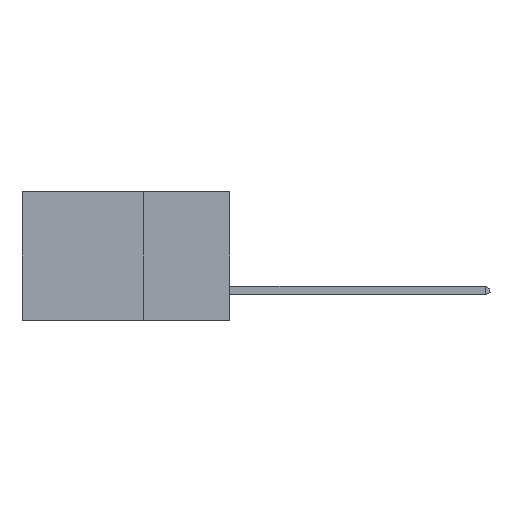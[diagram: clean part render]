
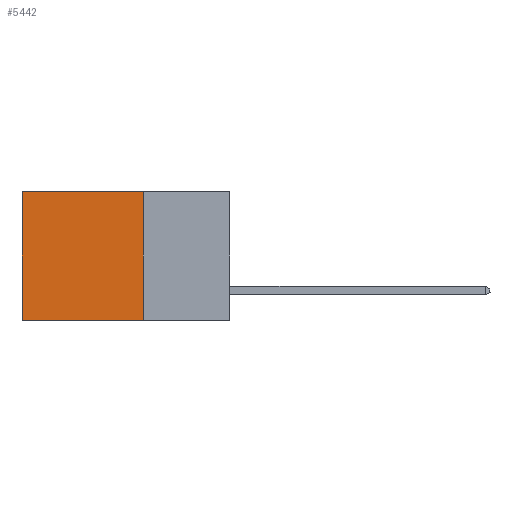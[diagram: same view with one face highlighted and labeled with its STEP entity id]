
A CAD part, left-side view. The second image highlights one B-rep face of the part: STEP entity #5442.
In plain terms, the highlighted planar face has unit normal (-1, 0, 0).
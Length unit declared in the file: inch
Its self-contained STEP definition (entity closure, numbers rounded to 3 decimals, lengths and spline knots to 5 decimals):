
#1410 = ORIENTED_EDGE ( 'NONE', *, *, #19259, .F. ) ;
#1640 = FACE_OUTER_BOUND ( 'NONE', #2733, .T. ) ;
#1818 = LINE ( 'NONE', #10269, #3425 ) ;
#2164 = VERTEX_POINT ( 'NONE', #7322 ) ;
#2174 = LINE ( 'NONE', #19444, #2698 ) ;
#2231 = ORIENTED_EDGE ( 'NONE', *, *, #9099, .T. ) ;
#2688 = PLANE ( 'NONE',  #17670 ) ;
#2698 = VECTOR ( 'NONE', #7493, 39.37008 ) ;
#2733 = EDGE_LOOP ( 'NONE', ( #9293, #13278, #1410, #2231 ) ) ;
#2766 = DIRECTION ( 'NONE',  ( 1., 0., 0. ) ) ;
#2942 = CARTESIAN_POINT ( 'NONE',  ( 0.298, 0.25, 0. ) ) ;
#3425 = VECTOR ( 'NONE', #22427, 39.37008 ) ;
#3997 = DIRECTION ( 'NONE',  ( 0., 1., 0. ) ) ;
#4279 = EDGE_CURVE ( 'NONE', #2164, #12227, #11445, .T. ) ;
#5243 = VECTOR ( 'NONE', #5940, 39.37008 ) ;
#5442 = ADVANCED_FACE ( 'NONE', ( #1640 ), #2688, .F. ) ;
#5940 = DIRECTION ( 'NONE',  ( 0., 1., 0. ) ) ;
#7322 = CARTESIAN_POINT ( 'NONE',  ( 0.298, 0.25, -0.37 ) ) ;
#7493 = DIRECTION ( 'NONE',  ( 0., 0., -1. ) ) ;
#9099 = EDGE_CURVE ( 'NONE', #9433, #19829, #12307, .T. ) ;
#9228 = CARTESIAN_POINT ( 'NONE',  ( 0.298, 0.6, 0. ) ) ;
#9293 = ORIENTED_EDGE ( 'NONE', *, *, #10940, .T. ) ;
#9433 = VERTEX_POINT ( 'NONE', #2942 ) ;
#10146 = CARTESIAN_POINT ( 'NONE',  ( 0.298, 0.6, -0.37 ) ) ;
#10269 = CARTESIAN_POINT ( 'NONE',  ( 0.298, 0.25, 0. ) ) ;
#10940 = EDGE_CURVE ( 'NONE', #19829, #12227, #2174, .T. ) ;
#11239 = CARTESIAN_POINT ( 'NONE',  ( 0.298, 0.25, 0. ) ) ;
#11445 = LINE ( 'NONE', #21309, #20142 ) ;
#12227 = VERTEX_POINT ( 'NONE', #10146 ) ;
#12307 = LINE ( 'NONE', #12435, #5243 ) ;
#12435 = CARTESIAN_POINT ( 'NONE',  ( 0.298, 0.25, 0. ) ) ;
#13278 = ORIENTED_EDGE ( 'NONE', *, *, #4279, .F. ) ;
#17670 = AXIS2_PLACEMENT_3D ( 'NONE', #11239, #2766, #19980 ) ;
#19259 = EDGE_CURVE ( 'NONE', #9433, #2164, #1818, .T. ) ;
#19444 = CARTESIAN_POINT ( 'NONE',  ( 0.298, 0.6, 0. ) ) ;
#19829 = VERTEX_POINT ( 'NONE', #9228 ) ;
#19980 = DIRECTION ( 'NONE',  ( 0., 0., -1. ) ) ;
#20142 = VECTOR ( 'NONE', #3997, 39.37008 ) ;
#21309 = CARTESIAN_POINT ( 'NONE',  ( 0.298, 0.25, -0.37 ) ) ;
#22427 = DIRECTION ( 'NONE',  ( 0., 0., -1. ) ) ;
